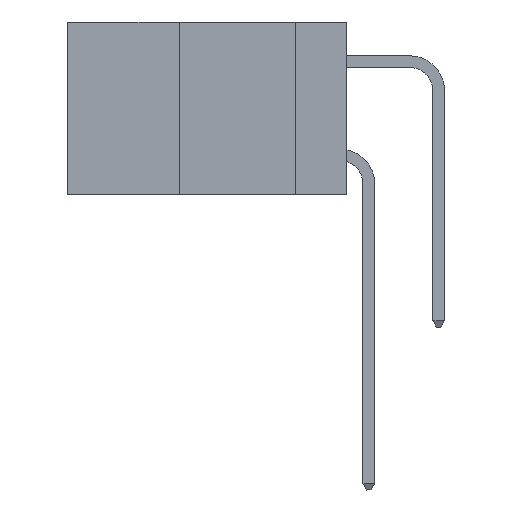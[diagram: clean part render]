
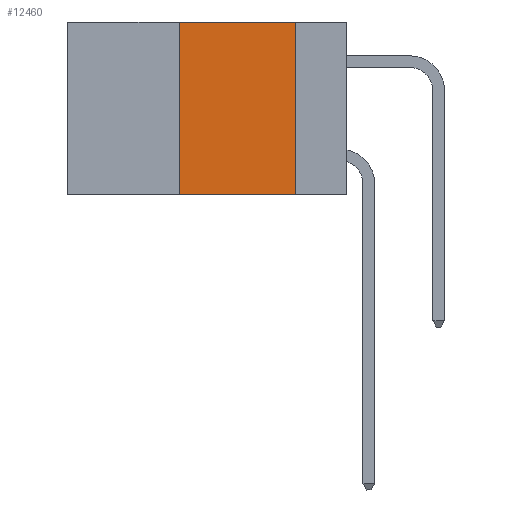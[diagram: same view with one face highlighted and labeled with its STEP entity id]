
A CAD part, left-side view. The second image highlights one B-rep face of the part: STEP entity #12460.
In plain terms, the highlighted planar face has unit normal (-1, 0, 0).
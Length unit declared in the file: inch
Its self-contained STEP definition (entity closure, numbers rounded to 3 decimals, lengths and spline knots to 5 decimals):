
#462 = DIRECTION ( 'NONE',  ( 0., -1., 0. ) ) ;
#2120 = LINE ( 'NONE', #17607, #20943 ) ;
#2355 = CARTESIAN_POINT ( 'NONE',  ( 0., 0.11, 0. ) ) ;
#2839 = LINE ( 'NONE', #22258, #12047 ) ;
#2886 = AXIS2_PLACEMENT_3D ( 'NONE', #13089, #14887, #3925 ) ;
#3688 = ORIENTED_EDGE ( 'NONE', *, *, #13812, .F. ) ;
#3745 = LINE ( 'NONE', #13062, #17203 ) ;
#3925 = DIRECTION ( 'NONE',  ( 0., 0., -1. ) ) ;
#4545 = ORIENTED_EDGE ( 'NONE', *, *, #22674, .F. ) ;
#4550 = VERTEX_POINT ( 'NONE', #20010 ) ;
#6636 = DIRECTION ( 'NONE',  ( 0., -1., 0. ) ) ;
#7320 = EDGE_CURVE ( 'NONE', #9386, #18964, #2120, .T. ) ;
#7977 = ORIENTED_EDGE ( 'NONE', *, *, #7320, .T. ) ;
#8588 = VECTOR ( 'NONE', #22106, 39.37008 ) ;
#9182 = LINE ( 'NONE', #16676, #8588 ) ;
#9386 = VERTEX_POINT ( 'NONE', #19394 ) ;
#9650 = EDGE_LOOP ( 'NONE', ( #3688, #4545, #16267, #7977 ) ) ;
#11251 = PLANE ( 'NONE',  #2886 ) ;
#12047 = VECTOR ( 'NONE', #462, 39.37008 ) ;
#12460 = ADVANCED_FACE ( 'NONE', ( #19169 ), #11251, .F. ) ;
#13062 = CARTESIAN_POINT ( 'NONE',  ( 0., 0.36, 0. ) ) ;
#13089 = CARTESIAN_POINT ( 'NONE',  ( 0., 0.6, 0. ) ) ;
#13812 = EDGE_CURVE ( 'NONE', #20742, #18964, #9182, .T. ) ;
#14862 = DIRECTION ( 'NONE',  ( 0., 0., 1. ) ) ;
#14887 = DIRECTION ( 'NONE',  ( 1., 0., 0. ) ) ;
#16267 = ORIENTED_EDGE ( 'NONE', *, *, #21967, .F. ) ;
#16676 = CARTESIAN_POINT ( 'NONE',  ( 0., 0.11, 0. ) ) ;
#17203 = VECTOR ( 'NONE', #14862, 39.37008 ) ;
#17607 = CARTESIAN_POINT ( 'NONE',  ( 0., 0.6, -0.37 ) ) ;
#18964 = VERTEX_POINT ( 'NONE', #21761 ) ;
#19169 = FACE_OUTER_BOUND ( 'NONE', #9650, .T. ) ;
#19394 = CARTESIAN_POINT ( 'NONE',  ( 0., 0.36, -0.37 ) ) ;
#20010 = CARTESIAN_POINT ( 'NONE',  ( 0., 0.36, 0. ) ) ;
#20742 = VERTEX_POINT ( 'NONE', #2355 ) ;
#20943 = VECTOR ( 'NONE', #6636, 39.37008 ) ;
#21761 = CARTESIAN_POINT ( 'NONE',  ( 0., 0.11, -0.37 ) ) ;
#21967 = EDGE_CURVE ( 'NONE', #9386, #4550, #3745, .T. ) ;
#22106 = DIRECTION ( 'NONE',  ( 0., 0., -1. ) ) ;
#22258 = CARTESIAN_POINT ( 'NONE',  ( 0., 0.6, 0. ) ) ;
#22674 = EDGE_CURVE ( 'NONE', #4550, #20742, #2839, .T. ) ;
